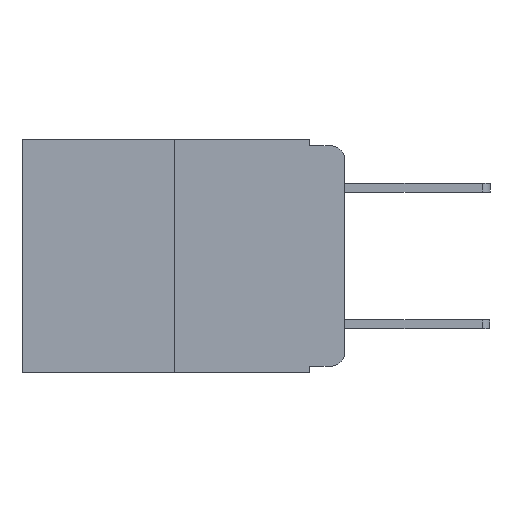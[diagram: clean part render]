
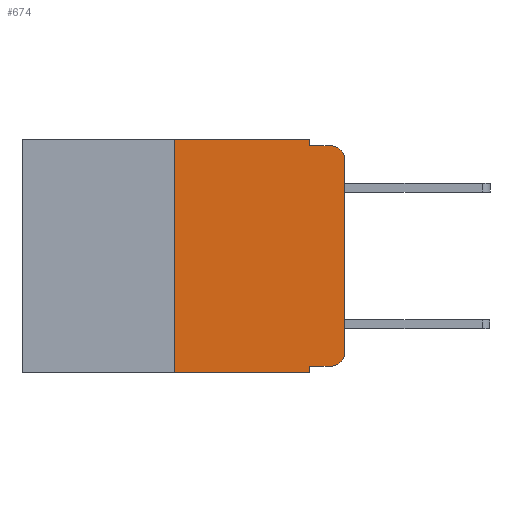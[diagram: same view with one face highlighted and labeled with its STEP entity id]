
A CAD part, left-side view. The second image highlights one B-rep face of the part: STEP entity #674.
In plain terms, the highlighted planar face has unit normal (-1, 0, 0).
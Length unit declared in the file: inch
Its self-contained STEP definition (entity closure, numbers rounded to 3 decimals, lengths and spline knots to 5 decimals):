
#208 = CARTESIAN_POINT ( 'NONE',  ( 0., 0.051, 0. ) ) ;
#285 = VECTOR ( 'NONE', #398, 39.37008 ) ;
#309 = LINE ( 'NONE', #8171, #673 ) ;
#398 = DIRECTION ( 'NONE',  ( 0., -1., 0. ) ) ;
#462 = ORIENTED_EDGE ( 'NONE', *, *, #8277, .T. ) ;
#498 = VERTEX_POINT ( 'NONE', #5747 ) ;
#673 = VECTOR ( 'NONE', #1736, 39.37008 ) ;
#674 = ADVANCED_FACE ( 'NONE', ( #8467 ), #12274, .F. ) ;
#686 = VERTEX_POINT ( 'NONE', #11291 ) ;
#934 = CARTESIAN_POINT ( 'NONE',  ( 0., 0.051, 0. ) ) ;
#1344 = LINE ( 'NONE', #12832, #12152 ) ;
#1360 = DIRECTION ( 'NONE',  ( 0., 0., -1. ) ) ;
#1433 = ORIENTED_EDGE ( 'NONE', *, *, #3595, .T. ) ;
#1539 = ORIENTED_EDGE ( 'NONE', *, *, #3670, .T. ) ;
#1565 = CARTESIAN_POINT ( 'NONE',  ( 0., 0., -0.03 ) ) ;
#1634 = ORIENTED_EDGE ( 'NONE', *, *, #4466, .F. ) ;
#1736 = DIRECTION ( 'NONE',  ( 0., -1., 0. ) ) ;
#2057 = DIRECTION ( 'NONE',  ( 1., 0., 0. ) ) ;
#2104 = LINE ( 'NONE', #208, #12484 ) ;
#2112 = DIRECTION ( 'NONE',  ( 0., 0., -1. ) ) ;
#2207 = AXIS2_PLACEMENT_3D ( 'NONE', #9706, #3450, #10674 ) ;
#2310 = CARTESIAN_POINT ( 'NONE',  ( 0., 0.473, 0. ) ) ;
#2708 = CARTESIAN_POINT ( 'NONE',  ( 0., 0.02, -0.313 ) ) ;
#2941 = CARTESIAN_POINT ( 'NONE',  ( 0., 0.051, -0.01 ) ) ;
#3040 = LINE ( 'NONE', #6062, #8314 ) ;
#3162 = CIRCLE ( 'NONE', #2207, 0.02 ) ;
#3352 = LINE ( 'NONE', #7965, #285 ) ;
#3418 = VERTEX_POINT ( 'NONE', #3531 ) ;
#3450 = DIRECTION ( 'NONE',  ( -1., 0., 0. ) ) ;
#3531 = CARTESIAN_POINT ( 'NONE',  ( 0., 0.25, 0. ) ) ;
#3595 = EDGE_CURVE ( 'NONE', #11767, #6124, #12820, .T. ) ;
#3670 = EDGE_CURVE ( 'NONE', #5314, #11767, #309, .T. ) ;
#3802 = DIRECTION ( 'NONE',  ( 0., 0., -1. ) ) ;
#4466 = EDGE_CURVE ( 'NONE', #5314, #7153, #12822, .T. ) ;
#5272 = EDGE_CURVE ( 'NONE', #9819, #3418, #5690, .T. ) ;
#5314 = VERTEX_POINT ( 'NONE', #9824 ) ;
#5334 = EDGE_CURVE ( 'NONE', #498, #9149, #2104, .T. ) ;
#5428 = EDGE_CURVE ( 'NONE', #9149, #686, #3352, .T. ) ;
#5690 = LINE ( 'NONE', #7649, #13393 ) ;
#5747 = CARTESIAN_POINT ( 'NONE',  ( 0., 0.051, 0. ) ) ;
#5947 = ORIENTED_EDGE ( 'NONE', *, *, #6306, .T. ) ;
#5970 = ORIENTED_EDGE ( 'NONE', *, *, #5334, .F. ) ;
#6062 = CARTESIAN_POINT ( 'NONE',  ( 0., 0.473, 0. ) ) ;
#6124 = VERTEX_POINT ( 'NONE', #13422 ) ;
#6225 = EDGE_CURVE ( 'NONE', #7840, #686, #3162, .T. ) ;
#6306 = EDGE_CURVE ( 'NONE', #6124, #7840, #1344, .T. ) ;
#6346 = DIRECTION ( 'NONE',  ( 0., 0., -1. ) ) ;
#6403 = CARTESIAN_POINT ( 'NONE',  ( 0., 0.02, -0.333 ) ) ;
#6820 = DIRECTION ( 'NONE',  ( 0., 0., 1. ) ) ;
#6861 = AXIS2_PLACEMENT_3D ( 'NONE', #2708, #10037, #3802 ) ;
#6887 = ORIENTED_EDGE ( 'NONE', *, *, #5272, .F. ) ;
#7153 = VERTEX_POINT ( 'NONE', #10030 ) ;
#7649 = CARTESIAN_POINT ( 'NONE',  ( 0., 0.25, 0. ) ) ;
#7672 = ORIENTED_EDGE ( 'NONE', *, *, #10116, .F. ) ;
#7840 = VERTEX_POINT ( 'NONE', #1565 ) ;
#7855 = DIRECTION ( 'NONE',  ( 0., -1., 0. ) ) ;
#7965 = CARTESIAN_POINT ( 'NONE',  ( 0., 0.051, -0.01 ) ) ;
#8054 = AXIS2_PLACEMENT_3D ( 'NONE', #2310, #2057, #6346 ) ;
#8118 = DIRECTION ( 'NONE',  ( 0., -1., 0. ) ) ;
#8171 = CARTESIAN_POINT ( 'NONE',  ( 0., 0.051, -0.333 ) ) ;
#8200 = ORIENTED_EDGE ( 'NONE', *, *, #6225, .T. ) ;
#8277 = EDGE_CURVE ( 'NONE', #9819, #7153, #11645, .T. ) ;
#8314 = VECTOR ( 'NONE', #8118, 39.37008 ) ;
#8467 = FACE_OUTER_BOUND ( 'NONE', #13538, .T. ) ;
#8665 = CARTESIAN_POINT ( 'NONE',  ( 0., 0.25, -0.343 ) ) ;
#9149 = VERTEX_POINT ( 'NONE', #2941 ) ;
#9706 = CARTESIAN_POINT ( 'NONE',  ( 0., 0.02, -0.03 ) ) ;
#9819 = VERTEX_POINT ( 'NONE', #8665 ) ;
#9824 = CARTESIAN_POINT ( 'NONE',  ( 0., 0.051, -0.333 ) ) ;
#9960 = ORIENTED_EDGE ( 'NONE', *, *, #5428, .F. ) ;
#10030 = CARTESIAN_POINT ( 'NONE',  ( 0., 0.051, -0.343 ) ) ;
#10037 = DIRECTION ( 'NONE',  ( -1., 0., 0. ) ) ;
#10116 = EDGE_CURVE ( 'NONE', #3418, #498, #3040, .T. ) ;
#10222 = VECTOR ( 'NONE', #2112, 39.37008 ) ;
#10287 = VECTOR ( 'NONE', #7855, 39.37008 ) ;
#10674 = DIRECTION ( 'NONE',  ( 0., 0., -1. ) ) ;
#11291 = CARTESIAN_POINT ( 'NONE',  ( 0., 0.02, -0.01 ) ) ;
#11645 = LINE ( 'NONE', #12834, #10287 ) ;
#11767 = VERTEX_POINT ( 'NONE', #6403 ) ;
#12152 = VECTOR ( 'NONE', #6820, 39.37008 ) ;
#12274 = PLANE ( 'NONE',  #8054 ) ;
#12484 = VECTOR ( 'NONE', #1360, 39.37008 ) ;
#12682 = DIRECTION ( 'NONE',  ( 0., 0., 1. ) ) ;
#12820 = CIRCLE ( 'NONE', #6861, 0.02 ) ;
#12822 = LINE ( 'NONE', #934, #10222 ) ;
#12832 = CARTESIAN_POINT ( 'NONE',  ( 0., 0., 0. ) ) ;
#12834 = CARTESIAN_POINT ( 'NONE',  ( 0., 0.473, -0.343 ) ) ;
#13393 = VECTOR ( 'NONE', #12682, 39.37008 ) ;
#13422 = CARTESIAN_POINT ( 'NONE',  ( 0., 0., -0.313 ) ) ;
#13538 = EDGE_LOOP ( 'NONE', ( #5947, #8200, #9960, #5970, #7672, #6887, #462, #1634, #1539, #1433 ) ) ;
